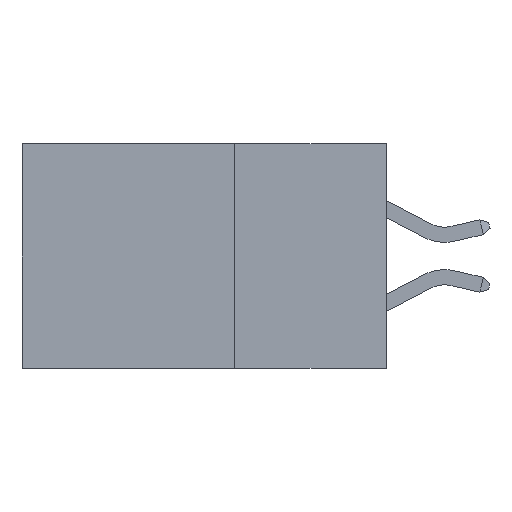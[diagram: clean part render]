
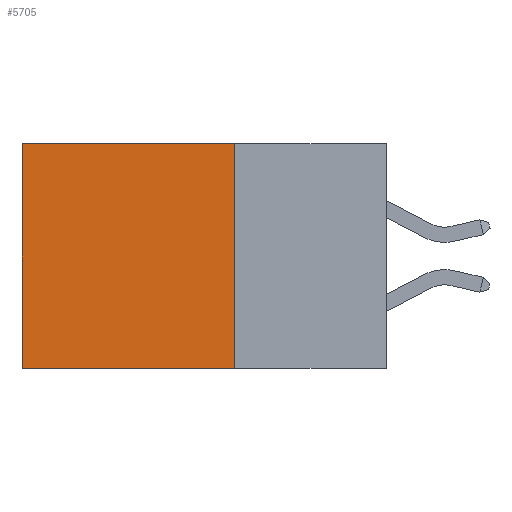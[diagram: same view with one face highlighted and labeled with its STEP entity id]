
A CAD part, left-side view. The second image highlights one B-rep face of the part: STEP entity #5705.
In plain terms, the highlighted planar face has unit normal (-1, 0, 0).
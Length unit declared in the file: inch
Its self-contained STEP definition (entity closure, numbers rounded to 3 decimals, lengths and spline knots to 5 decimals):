
#1399 = VECTOR ( 'NONE', #12320, 39.37008 ) ;
#2481 = ORIENTED_EDGE ( 'NONE', *, *, #15218, .T. ) ;
#2841 = DIRECTION ( 'NONE',  ( 0., 1., 0. ) ) ;
#3082 = CARTESIAN_POINT ( 'NONE',  ( 0.2615, 0.25, -0.37 ) ) ;
#3205 = EDGE_CURVE ( 'NONE', #7391, #8838, #7322, .T. ) ;
#3386 = AXIS2_PLACEMENT_3D ( 'NONE', #12632, #14195, #14031 ) ;
#3403 = VECTOR ( 'NONE', #2841, 39.37008 ) ;
#4150 = CARTESIAN_POINT ( 'NONE',  ( 0.2615, 0.6, 0. ) ) ;
#4356 = ORIENTED_EDGE ( 'NONE', *, *, #11768, .T. ) ;
#4733 = CARTESIAN_POINT ( 'NONE',  ( 0.2615, 0.25, -0.37 ) ) ;
#5682 = VECTOR ( 'NONE', #6303, 39.37008 ) ;
#5705 = ADVANCED_FACE ( 'NONE', ( #7949 ), #12945, .F. ) ;
#5709 = CARTESIAN_POINT ( 'NONE',  ( 0.2615, 0.25, 0. ) ) ;
#6303 = DIRECTION ( 'NONE',  ( 0., 0., -1. ) ) ;
#6618 = CARTESIAN_POINT ( 'NONE',  ( 0.2615, 0.6, -0.37 ) ) ;
#7322 = LINE ( 'NONE', #4733, #1399 ) ;
#7391 = VERTEX_POINT ( 'NONE', #14853 ) ;
#7777 = LINE ( 'NONE', #12694, #3403 ) ;
#7949 = FACE_OUTER_BOUND ( 'NONE', #9356, .T. ) ;
#8065 = LINE ( 'NONE', #5709, #9779 ) ;
#8332 = ORIENTED_EDGE ( 'NONE', *, *, #9493, .F. ) ;
#8358 = ORIENTED_EDGE ( 'NONE', *, *, #3205, .F. ) ;
#8664 = LINE ( 'NONE', #11209, #5682 ) ;
#8838 = VERTEX_POINT ( 'NONE', #3082 ) ;
#9356 = EDGE_LOOP ( 'NONE', ( #2481, #8332, #8358, #4356 ) ) ;
#9493 = EDGE_CURVE ( 'NONE', #8838, #15360, #7777, .T. ) ;
#9779 = VECTOR ( 'NONE', #11990, 39.37008 ) ;
#11209 = CARTESIAN_POINT ( 'NONE',  ( 0.2615, 0.6, -0.37 ) ) ;
#11768 = EDGE_CURVE ( 'NONE', #7391, #14464, #8065, .T. ) ;
#11990 = DIRECTION ( 'NONE',  ( 0., 1., 0. ) ) ;
#12320 = DIRECTION ( 'NONE',  ( 0., 0., -1. ) ) ;
#12632 = CARTESIAN_POINT ( 'NONE',  ( 0.2615, 0.25, -0.37 ) ) ;
#12694 = CARTESIAN_POINT ( 'NONE',  ( 0.2615, 0.25, -0.37 ) ) ;
#12945 = PLANE ( 'NONE',  #3386 ) ;
#14031 = DIRECTION ( 'NONE',  ( 0., 0., -1. ) ) ;
#14195 = DIRECTION ( 'NONE',  ( 1., 0., 0. ) ) ;
#14464 = VERTEX_POINT ( 'NONE', #4150 ) ;
#14853 = CARTESIAN_POINT ( 'NONE',  ( 0.2615, 0.25, 0. ) ) ;
#15218 = EDGE_CURVE ( 'NONE', #14464, #15360, #8664, .T. ) ;
#15360 = VERTEX_POINT ( 'NONE', #6618 ) ;
